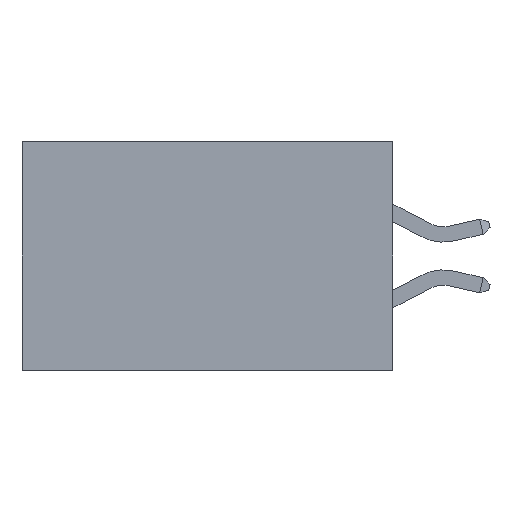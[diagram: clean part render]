
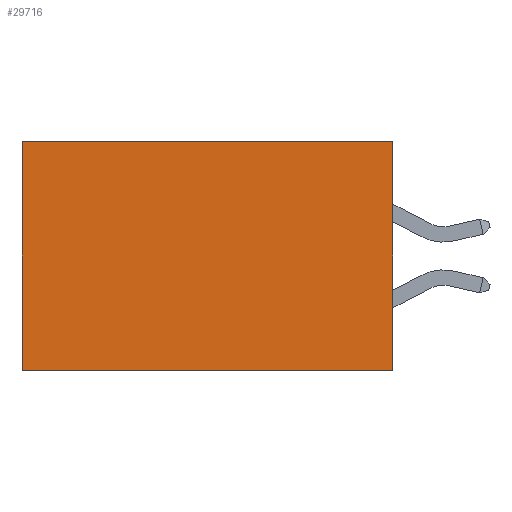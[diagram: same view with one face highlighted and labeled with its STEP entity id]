
A CAD part, left-side view. The second image highlights one B-rep face of the part: STEP entity #29716.
In plain terms, the highlighted planar face has unit normal (-1, 0, 0).
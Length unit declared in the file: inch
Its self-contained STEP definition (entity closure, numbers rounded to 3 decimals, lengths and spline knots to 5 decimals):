
#385 = LINE ( 'NONE', #2528, #27885 ) ;
#856 = EDGE_LOOP ( 'NONE', ( #23845, #28910, #28801, #7623 ) ) ;
#1121 = DIRECTION ( 'NONE',  ( 1., 0., 0. ) ) ;
#1165 = DIRECTION ( 'NONE',  ( 0., 0., -1. ) ) ;
#2528 = CARTESIAN_POINT ( 'NONE',  ( 0.2875, 0.6, 0. ) ) ;
#3385 = LINE ( 'NONE', #10805, #7958 ) ;
#4993 = CARTESIAN_POINT ( 'NONE',  ( 0.2875, 0., -0.37 ) ) ;
#6172 = CARTESIAN_POINT ( 'NONE',  ( 0.2875, 0., 0. ) ) ;
#6995 = VECTOR ( 'NONE', #19161, 39.37008 ) ;
#7317 = EDGE_CURVE ( 'NONE', #20390, #18775, #385, .T. ) ;
#7623 = ORIENTED_EDGE ( 'NONE', *, *, #16495, .T. ) ;
#7761 = VECTOR ( 'NONE', #1165, 39.37008 ) ;
#7958 = VECTOR ( 'NONE', #18179, 39.37008 ) ;
#8212 = EDGE_CURVE ( 'NONE', #28804, #18775, #3385, .T. ) ;
#9457 = AXIS2_PLACEMENT_3D ( 'NONE', #11899, #1121, #29375 ) ;
#10805 = CARTESIAN_POINT ( 'NONE',  ( 0.2875, 0., -0.37 ) ) ;
#11136 = EDGE_CURVE ( 'NONE', #31527, #28804, #20362, .T. ) ;
#11899 = CARTESIAN_POINT ( 'NONE',  ( 0.2875, 0., 0. ) ) ;
#13911 = FACE_OUTER_BOUND ( 'NONE', #856, .T. ) ;
#13984 = CARTESIAN_POINT ( 'NONE',  ( 0.2875, 0.6, 0. ) ) ;
#14086 = CARTESIAN_POINT ( 'NONE',  ( 0.2875, 0., 0. ) ) ;
#16378 = CARTESIAN_POINT ( 'NONE',  ( 0.2875, 0., 0. ) ) ;
#16495 = EDGE_CURVE ( 'NONE', #31527, #20390, #26843, .T. ) ;
#18179 = DIRECTION ( 'NONE',  ( 0., 1., 0. ) ) ;
#18775 = VERTEX_POINT ( 'NONE', #22098 ) ;
#19161 = DIRECTION ( 'NONE',  ( 0., 1., 0. ) ) ;
#20362 = LINE ( 'NONE', #6172, #7761 ) ;
#20390 = VERTEX_POINT ( 'NONE', #13984 ) ;
#22098 = CARTESIAN_POINT ( 'NONE',  ( 0.2875, 0.6, -0.37 ) ) ;
#23845 = ORIENTED_EDGE ( 'NONE', *, *, #7317, .T. ) ;
#26843 = LINE ( 'NONE', #16378, #6995 ) ;
#27154 = DIRECTION ( 'NONE',  ( 0., 0., -1. ) ) ;
#27885 = VECTOR ( 'NONE', #27154, 39.37008 ) ;
#27936 = PLANE ( 'NONE',  #9457 ) ;
#28801 = ORIENTED_EDGE ( 'NONE', *, *, #11136, .F. ) ;
#28804 = VERTEX_POINT ( 'NONE', #4993 ) ;
#28910 = ORIENTED_EDGE ( 'NONE', *, *, #8212, .F. ) ;
#29375 = DIRECTION ( 'NONE',  ( 0., 0., -1. ) ) ;
#29716 = ADVANCED_FACE ( 'NONE', ( #13911 ), #27936, .F. ) ;
#31527 = VERTEX_POINT ( 'NONE', #14086 ) ;
